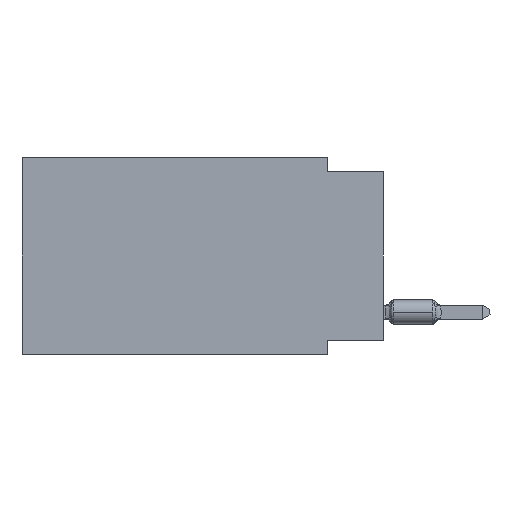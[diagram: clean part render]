
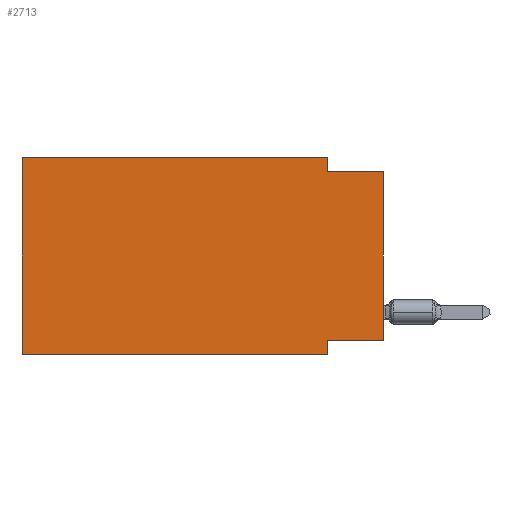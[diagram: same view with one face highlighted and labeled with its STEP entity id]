
A CAD part, left-side view. The second image highlights one B-rep face of the part: STEP entity #2713.
In plain terms, the highlighted planar face has unit normal (-1, 0, 0).
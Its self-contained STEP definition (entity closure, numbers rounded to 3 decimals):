
#95 = CARTESIAN_POINT ( 'NONE',  ( 0., 2.54, -8.255 ) ) ;
#123 = ORIENTED_EDGE ( 'NONE', *, *, #25321, .F. ) ;
#776 = ORIENTED_EDGE ( 'NONE', *, *, #10458, .T. ) ;
#1769 = CARTESIAN_POINT ( 'NONE',  ( 0., 2.54, 0. ) ) ;
#1987 = DIRECTION ( 'NONE',  ( 0., 0., 1. ) ) ;
#2400 = LINE ( 'NONE', #12696, #24314 ) ;
#2713 = ADVANCED_FACE ( 'NONE', ( #6287 ), #23894, .F. ) ;
#3220 = CARTESIAN_POINT ( 'NONE',  ( 0., 16.383, 0. ) ) ;
#3578 = DIRECTION ( 'NONE',  ( 0., 0., -1. ) ) ;
#3607 = VECTOR ( 'NONE', #14179, 1000. ) ;
#3738 = CARTESIAN_POINT ( 'NONE',  ( 0., 16.383, 0. ) ) ;
#3797 = ORIENTED_EDGE ( 'NONE', *, *, #21399, .F. ) ;
#4219 = DIRECTION ( 'NONE',  ( 0., 0., -1. ) ) ;
#4548 = CARTESIAN_POINT ( 'NONE',  ( 0., 0., -0.635 ) ) ;
#5743 = CARTESIAN_POINT ( 'NONE',  ( 0., 2.54, -8.89 ) ) ;
#6287 = FACE_OUTER_BOUND ( 'NONE', #9205, .T. ) ;
#6312 = VERTEX_POINT ( 'NONE', #22605 ) ;
#6340 = VECTOR ( 'NONE', #1987, 1000. ) ;
#6563 = DIRECTION ( 'NONE',  ( 0., -1., 0. ) ) ;
#6716 = VERTEX_POINT ( 'NONE', #13796 ) ;
#6842 = ORIENTED_EDGE ( 'NONE', *, *, #12191, .F. ) ;
#7982 = ORIENTED_EDGE ( 'NONE', *, *, #18475, .F. ) ;
#9205 = EDGE_LOOP ( 'NONE', ( #20372, #3797, #6842, #24658, #7982, #776, #123, #22120 ) ) ;
#9328 = VERTEX_POINT ( 'NONE', #95 ) ;
#10052 = VECTOR ( 'NONE', #3578, 1000. ) ;
#10213 = VECTOR ( 'NONE', #6563, 1000. ) ;
#10298 = LINE ( 'NONE', #18648, #10213 ) ;
#10458 = EDGE_CURVE ( 'NONE', #21621, #17080, #10298, .T. ) ;
#11133 = LINE ( 'NONE', #19103, #19026 ) ;
#11490 = CARTESIAN_POINT ( 'NONE',  ( 0., 16.383, -8.89 ) ) ;
#11626 = VECTOR ( 'NONE', #21907, 1000. ) ;
#11771 = CARTESIAN_POINT ( 'NONE',  ( 0., 16.383, 0. ) ) ;
#12191 = EDGE_CURVE ( 'NONE', #6716, #22652, #19393, .T. ) ;
#12207 = CARTESIAN_POINT ( 'NONE',  ( 0., 16.383, 0. ) ) ;
#12696 = CARTESIAN_POINT ( 'NONE',  ( 0., 0., -8.255 ) ) ;
#12842 = VERTEX_POINT ( 'NONE', #4548 ) ;
#13537 = LINE ( 'NONE', #17395, #15565 ) ;
#13796 = CARTESIAN_POINT ( 'NONE',  ( 0., 2.54, 0. ) ) ;
#14179 = DIRECTION ( 'NONE',  ( 0., -1., 0. ) ) ;
#15565 = VECTOR ( 'NONE', #21000, 1000. ) ;
#16549 = DIRECTION ( 'NONE',  ( 0., 1., 0. ) ) ;
#17080 = VERTEX_POINT ( 'NONE', #5743 ) ;
#17395 = CARTESIAN_POINT ( 'NONE',  ( 0., 2.54, -8.89 ) ) ;
#18475 = EDGE_CURVE ( 'NONE', #21621, #19830, #23463, .T. ) ;
#18648 = CARTESIAN_POINT ( 'NONE',  ( 0., 16.383, -8.89 ) ) ;
#19026 = VECTOR ( 'NONE', #23077, 1000. ) ;
#19103 = CARTESIAN_POINT ( 'NONE',  ( 0., 0., -0.635 ) ) ;
#19393 = LINE ( 'NONE', #1769, #10052 ) ;
#19830 = VERTEX_POINT ( 'NONE', #3220 ) ;
#19960 = LINE ( 'NONE', #3738, #3607 ) ;
#20372 = ORIENTED_EDGE ( 'NONE', *, *, #21846, .T. ) ;
#20499 = EDGE_CURVE ( 'NONE', #6312, #9328, #2400, .T. ) ;
#21000 = DIRECTION ( 'NONE',  ( 0., 0., -1. ) ) ;
#21399 = EDGE_CURVE ( 'NONE', #22652, #12842, #11133, .T. ) ;
#21621 = VERTEX_POINT ( 'NONE', #11490 ) ;
#21846 = EDGE_CURVE ( 'NONE', #6312, #12842, #23828, .T. ) ;
#21907 = DIRECTION ( 'NONE',  ( 0., 0., 1. ) ) ;
#22120 = ORIENTED_EDGE ( 'NONE', *, *, #20499, .F. ) ;
#22193 = CARTESIAN_POINT ( 'NONE',  ( 0., 2.54, -0.635 ) ) ;
#22605 = CARTESIAN_POINT ( 'NONE',  ( 0., 0., -8.255 ) ) ;
#22652 = VERTEX_POINT ( 'NONE', #22193 ) ;
#23077 = DIRECTION ( 'NONE',  ( 0., -1., 0. ) ) ;
#23463 = LINE ( 'NONE', #11771, #6340 ) ;
#23475 = AXIS2_PLACEMENT_3D ( 'NONE', #12207, #25447, #4219 ) ;
#23828 = LINE ( 'NONE', #23951, #11626 ) ;
#23894 = PLANE ( 'NONE',  #23475 ) ;
#23951 = CARTESIAN_POINT ( 'NONE',  ( 0., 0., 0. ) ) ;
#24203 = EDGE_CURVE ( 'NONE', #19830, #6716, #19960, .T. ) ;
#24314 = VECTOR ( 'NONE', #16549, 1000. ) ;
#24658 = ORIENTED_EDGE ( 'NONE', *, *, #24203, .F. ) ;
#25321 = EDGE_CURVE ( 'NONE', #9328, #17080, #13537, .T. ) ;
#25447 = DIRECTION ( 'NONE',  ( 1., 0., 0. ) ) ;
